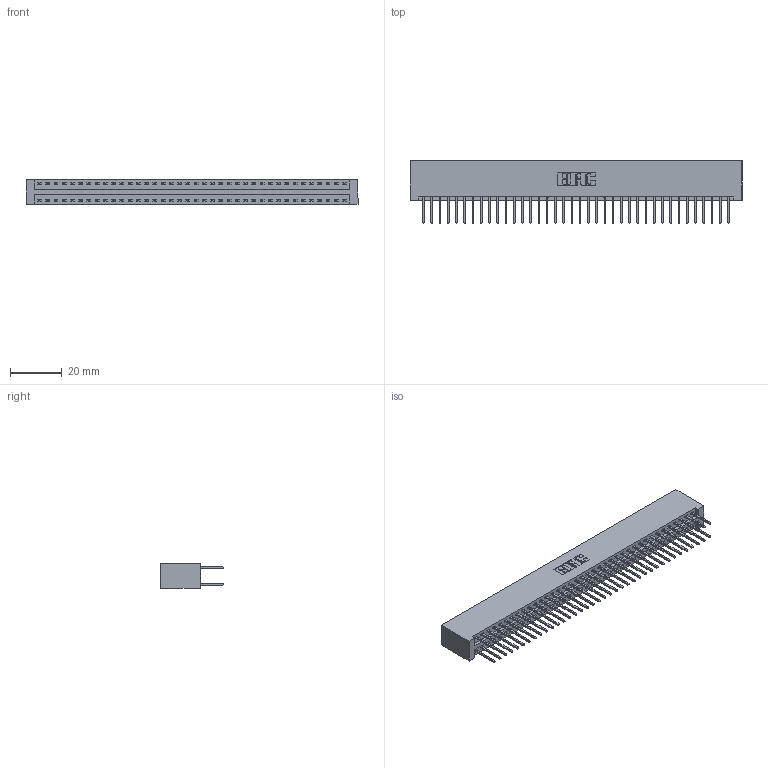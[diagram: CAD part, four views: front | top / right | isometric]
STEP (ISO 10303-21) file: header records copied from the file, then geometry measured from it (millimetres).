
FILE_DESCRIPTION (( 'STEP AP203' ), '1' );
FILE_NAME ('396-076-526-201.STEP', '2018-09-09T13:37:09', ( '' ), ( '' ), 'SwSTEP 2.0', 'SolidWorks 2016', '' );
FILE_SCHEMA (( 'CONFIG_CONTROL_DESIGN' ));
Length unit declared in the file: inch
Products named in the file (3): 345-292-001_345-293-126; 396-076-526-201; 346 Part_No Mounting Lugs
Assembly tree (77 placements, depth 2):
  396-076-526-201
    346 Part_No Mounting Lugs
    345-292-001_345-293-126  x76
Bounding box: 127.89 x 24.13 x 9.4 mm (x, y, z)
Volume: 13137.6 mm3; surface area: 18716.7 mm2
Topology: 77 solids, 77 shells, 4066 faces, 12085 edges, 7954 vertices
Faces by surface type: plane 2732, cylinder 1334
Entity records: 25079 total; most frequent: CARTESIAN_POINT 4136, ORIENTED_EDGE 4070, DIRECTION 3691, EDGE_CURVE 2035, VECTOR 1759, LINE 1759, VERTEX_POINT 1354, AXIS2_PLACEMENT_3D 966
